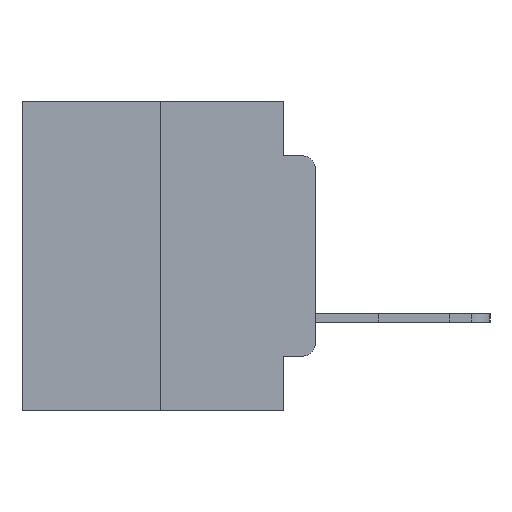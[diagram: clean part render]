
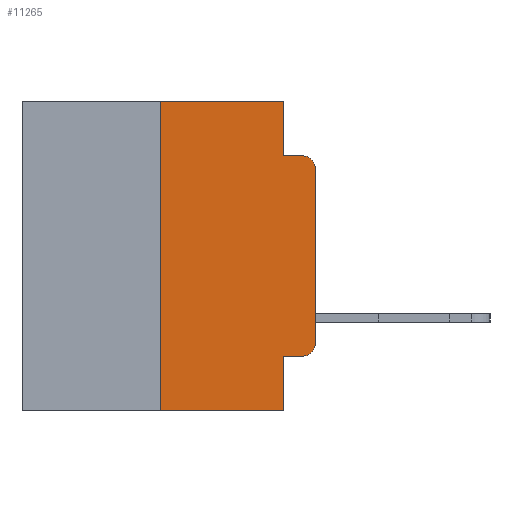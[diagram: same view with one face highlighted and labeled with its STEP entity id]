
A CAD part, left-side view. The second image highlights one B-rep face of the part: STEP entity #11265.
In plain terms, the highlighted planar face has unit normal (-1, 0, 0).
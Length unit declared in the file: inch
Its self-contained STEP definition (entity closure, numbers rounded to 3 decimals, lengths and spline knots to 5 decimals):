
#53 = CARTESIAN_POINT ( 'NONE',  ( 0., 0.25, -0.5 ) ) ;
#285 = LINE ( 'NONE', #9352, #20903 ) ;
#293 = CIRCLE ( 'NONE', #22791, 0.02 ) ;
#303 = ORIENTED_EDGE ( 'NONE', *, *, #902, .F. ) ;
#514 = CARTESIAN_POINT ( 'NONE',  ( 0., 0.051, 0. ) ) ;
#561 = LINE ( 'NONE', #514, #25402 ) ;
#591 = EDGE_CURVE ( 'NONE', #20662, #12032, #1904, .T. ) ;
#767 = ORIENTED_EDGE ( 'NONE', *, *, #6909, .F. ) ;
#902 = EDGE_CURVE ( 'NONE', #11221, #7099, #7257, .T. ) ;
#909 = DIRECTION ( 'NONE',  ( 0., 0., -1. ) ) ;
#1469 = DIRECTION ( 'NONE',  ( 0., 0., -1. ) ) ;
#1834 = VECTOR ( 'NONE', #18406, 39.37008 ) ;
#1904 = LINE ( 'NONE', #11354, #16774 ) ;
#2526 = LINE ( 'NONE', #20252, #1834 ) ;
#2746 = DIRECTION ( 'NONE',  ( 0., -1., 0. ) ) ;
#2971 = ORIENTED_EDGE ( 'NONE', *, *, #19415, .T. ) ;
#2990 = EDGE_CURVE ( 'NONE', #21508, #24588, #13348, .T. ) ;
#3425 = DIRECTION ( 'NONE',  ( 0., -1., 0. ) ) ;
#3880 = FACE_OUTER_BOUND ( 'NONE', #7427, .T. ) ;
#4162 = ORIENTED_EDGE ( 'NONE', *, *, #23132, .T. ) ;
#4889 = CARTESIAN_POINT ( 'NONE',  ( 0., 0.051, -0.0885 ) ) ;
#5142 = ORIENTED_EDGE ( 'NONE', *, *, #2990, .F. ) ;
#5698 = ORIENTED_EDGE ( 'NONE', *, *, #25188, .T. ) ;
#5930 = DIRECTION ( 'NONE',  ( 1., 0., 0. ) ) ;
#6047 = CARTESIAN_POINT ( 'NONE',  ( 0., 0.02, -0.0885 ) ) ;
#6131 = ORIENTED_EDGE ( 'NONE', *, *, #14771, .T. ) ;
#6623 = VECTOR ( 'NONE', #3425, 39.37008 ) ;
#6902 = CARTESIAN_POINT ( 'NONE',  ( 0., 0.473, 0. ) ) ;
#6909 = EDGE_CURVE ( 'NONE', #13414, #11221, #285, .T. ) ;
#6929 = DIRECTION ( 'NONE',  ( 0., 0., -1. ) ) ;
#7011 = ORIENTED_EDGE ( 'NONE', *, *, #9695, .F. ) ;
#7099 = VERTEX_POINT ( 'NONE', #19423 ) ;
#7257 = LINE ( 'NONE', #6902, #10121 ) ;
#7427 = EDGE_LOOP ( 'NONE', ( #2971, #4162, #5142, #7011, #303, #767, #5698, #9699, #11023, #6131 ) ) ;
#7628 = CARTESIAN_POINT ( 'NONE',  ( 0., 0.473, -0.5 ) ) ;
#9352 = CARTESIAN_POINT ( 'NONE',  ( 0., 0.25, 0. ) ) ;
#9410 = VERTEX_POINT ( 'NONE', #12060 ) ;
#9641 = DIRECTION ( 'NONE',  ( 0., 0., 1. ) ) ;
#9695 = EDGE_CURVE ( 'NONE', #7099, #21508, #561, .T. ) ;
#9699 = ORIENTED_EDGE ( 'NONE', *, *, #591, .F. ) ;
#10121 = VECTOR ( 'NONE', #2746, 39.37008 ) ;
#10263 = VERTEX_POINT ( 'NONE', #20250 ) ;
#11009 = AXIS2_PLACEMENT_3D ( 'NONE', #24454, #13296, #909 ) ;
#11023 = ORIENTED_EDGE ( 'NONE', *, *, #19812, .T. ) ;
#11221 = VERTEX_POINT ( 'NONE', #23119 ) ;
#11265 = ADVANCED_FACE ( 'NONE', ( #3880 ), #13885, .F. ) ;
#11354 = CARTESIAN_POINT ( 'NONE',  ( 0., 0.051, 0. ) ) ;
#12032 = VERTEX_POINT ( 'NONE', #21813 ) ;
#12060 = CARTESIAN_POINT ( 'NONE',  ( 0., 0., -0.1085 ) ) ;
#12250 = VECTOR ( 'NONE', #9641, 39.37008 ) ;
#12626 = LINE ( 'NONE', #7628, #6623 ) ;
#13264 = CIRCLE ( 'NONE', #11009, 0.02 ) ;
#13296 = DIRECTION ( 'NONE',  ( -1., 0., 0. ) ) ;
#13348 = LINE ( 'NONE', #21048, #18397 ) ;
#13414 = VERTEX_POINT ( 'NONE', #53 ) ;
#13782 = DIRECTION ( 'NONE',  ( -1., 0., 0. ) ) ;
#13885 = PLANE ( 'NONE',  #20276 ) ;
#14771 = EDGE_CURVE ( 'NONE', #10263, #21201, #293, .T. ) ;
#15826 = CARTESIAN_POINT ( 'NONE',  ( 0., 0.473, 0. ) ) ;
#16774 = VECTOR ( 'NONE', #19339, 39.37008 ) ;
#17332 = LINE ( 'NONE', #19063, #12250 ) ;
#17930 = CARTESIAN_POINT ( 'NONE',  ( 0., 0., -0.3915 ) ) ;
#18397 = VECTOR ( 'NONE', #20908, 39.37008 ) ;
#18406 = DIRECTION ( 'NONE',  ( 0., -1., 0. ) ) ;
#19063 = CARTESIAN_POINT ( 'NONE',  ( 0., 0., 0. ) ) ;
#19339 = DIRECTION ( 'NONE',  ( 0., 0., -1. ) ) ;
#19415 = EDGE_CURVE ( 'NONE', #21201, #9410, #17332, .T. ) ;
#19423 = CARTESIAN_POINT ( 'NONE',  ( 0., 0.051, 0. ) ) ;
#19561 = DIRECTION ( 'NONE',  ( 0., 0., -1. ) ) ;
#19812 = EDGE_CURVE ( 'NONE', #20662, #10263, #2526, .T. ) ;
#20133 = CARTESIAN_POINT ( 'NONE',  ( 0., 0.051, -0.4115 ) ) ;
#20250 = CARTESIAN_POINT ( 'NONE',  ( 0., 0.02, -0.4115 ) ) ;
#20252 = CARTESIAN_POINT ( 'NONE',  ( 0., 0.051, -0.4115 ) ) ;
#20276 = AXIS2_PLACEMENT_3D ( 'NONE', #15826, #5930, #19561 ) ;
#20662 = VERTEX_POINT ( 'NONE', #20133 ) ;
#20903 = VECTOR ( 'NONE', #24412, 39.37008 ) ;
#20908 = DIRECTION ( 'NONE',  ( 0., -1., 0. ) ) ;
#21048 = CARTESIAN_POINT ( 'NONE',  ( 0., 0.051, -0.0885 ) ) ;
#21201 = VERTEX_POINT ( 'NONE', #17930 ) ;
#21508 = VERTEX_POINT ( 'NONE', #4889 ) ;
#21813 = CARTESIAN_POINT ( 'NONE',  ( 0., 0.051, -0.5 ) ) ;
#22791 = AXIS2_PLACEMENT_3D ( 'NONE', #24919, #13782, #1469 ) ;
#23119 = CARTESIAN_POINT ( 'NONE',  ( 0., 0.25, 0. ) ) ;
#23132 = EDGE_CURVE ( 'NONE', #9410, #24588, #13264, .T. ) ;
#24412 = DIRECTION ( 'NONE',  ( 0., 0., 1. ) ) ;
#24454 = CARTESIAN_POINT ( 'NONE',  ( 0., 0.02, -0.1085 ) ) ;
#24588 = VERTEX_POINT ( 'NONE', #6047 ) ;
#24919 = CARTESIAN_POINT ( 'NONE',  ( 0., 0.02, -0.3915 ) ) ;
#25188 = EDGE_CURVE ( 'NONE', #13414, #12032, #12626, .T. ) ;
#25402 = VECTOR ( 'NONE', #6929, 39.37008 ) ;
